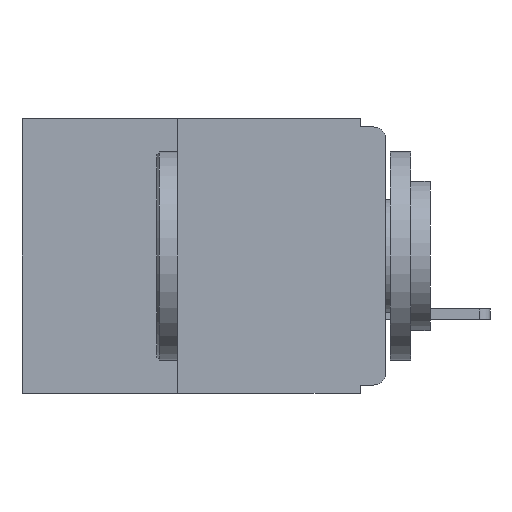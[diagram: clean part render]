
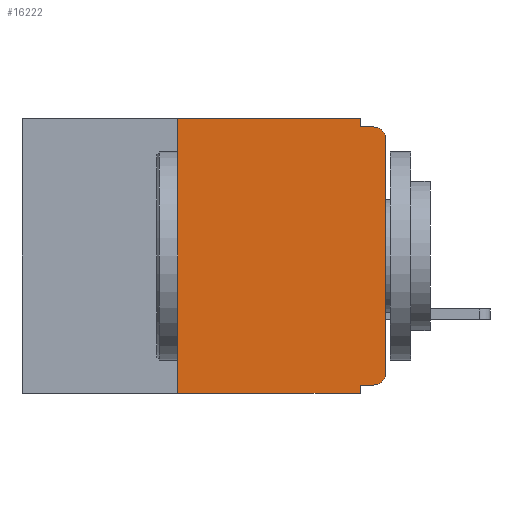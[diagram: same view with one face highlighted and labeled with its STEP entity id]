
A CAD part, left-side view. The second image highlights one B-rep face of the part: STEP entity #16222.
In plain terms, the highlighted planar face has unit normal (-1, 0, 0).
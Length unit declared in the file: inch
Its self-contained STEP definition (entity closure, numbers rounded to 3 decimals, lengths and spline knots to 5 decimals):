
#193 = CARTESIAN_POINT ( 'NONE',  ( 0., 0.25, -0.33 ) ) ;
#539 = VERTEX_POINT ( 'NONE', #2315 ) ;
#827 = DIRECTION ( 'NONE',  ( 0., 0., 1. ) ) ;
#1279 = VERTEX_POINT ( 'NONE', #30754 ) ;
#1551 = CARTESIAN_POINT ( 'NONE',  ( 0., 0.437, 0. ) ) ;
#1604 = VECTOR ( 'NONE', #6091, 39.37008 ) ;
#2132 = CARTESIAN_POINT ( 'NONE',  ( 0., 0., -0.025 ) ) ;
#2315 = CARTESIAN_POINT ( 'NONE',  ( 0., 0.031, -0.33 ) ) ;
#2567 = VERTEX_POINT ( 'NONE', #16467 ) ;
#2939 = ORIENTED_EDGE ( 'NONE', *, *, #4405, .F. ) ;
#4150 = DIRECTION ( 'NONE',  ( 0., -1., 0. ) ) ;
#4205 = LINE ( 'NONE', #1551, #23643 ) ;
#4405 = EDGE_CURVE ( 'NONE', #2567, #15590, #22816, .T. ) ;
#4991 = ORIENTED_EDGE ( 'NONE', *, *, #16368, .T. ) ;
#5085 = CARTESIAN_POINT ( 'NONE',  ( 0., 0.015, -0.305 ) ) ;
#5114 = VECTOR ( 'NONE', #10338, 39.37008 ) ;
#6091 = DIRECTION ( 'NONE',  ( 0., 0., -1. ) ) ;
#6800 = AXIS2_PLACEMENT_3D ( 'NONE', #28515, #13353, #31026 ) ;
#7520 = CARTESIAN_POINT ( 'NONE',  ( 0., 0.015, -0.32 ) ) ;
#7654 = DIRECTION ( 'NONE',  ( 0., 0., -1. ) ) ;
#7661 = ORIENTED_EDGE ( 'NONE', *, *, #28805, .F. ) ;
#7833 = VECTOR ( 'NONE', #26957, 39.37008 ) ;
#9112 = ORIENTED_EDGE ( 'NONE', *, *, #11240, .T. ) ;
#9179 = ORIENTED_EDGE ( 'NONE', *, *, #23349, .T. ) ;
#9200 = LINE ( 'NONE', #13595, #1604 ) ;
#10338 = DIRECTION ( 'NONE',  ( 0., 1., 0. ) ) ;
#10915 = AXIS2_PLACEMENT_3D ( 'NONE', #14170, #31842, #16793 ) ;
#11141 = CARTESIAN_POINT ( 'NONE',  ( 0., 0.031, -0.01 ) ) ;
#11240 = EDGE_CURVE ( 'NONE', #19077, #22179, #11876, .T. ) ;
#11675 = EDGE_CURVE ( 'NONE', #15250, #22444, #25360, .T. ) ;
#11876 = LINE ( 'NONE', #13205, #24597 ) ;
#11890 = ORIENTED_EDGE ( 'NONE', *, *, #26923, .F. ) ;
#12312 = DIRECTION ( 'NONE',  ( 0., -1., 0. ) ) ;
#12396 = EDGE_CURVE ( 'NONE', #22179, #15454, #22551, .T. ) ;
#12964 = LINE ( 'NONE', #19940, #31514 ) ;
#13205 = CARTESIAN_POINT ( 'NONE',  ( 0., 0., 0. ) ) ;
#13302 = EDGE_CURVE ( 'NONE', #15590, #15454, #14511, .T. ) ;
#13353 = DIRECTION ( 'NONE',  ( -1., 0., 0. ) ) ;
#13478 = CARTESIAN_POINT ( 'NONE',  ( 0., 0.25, -0.33 ) ) ;
#13595 = CARTESIAN_POINT ( 'NONE',  ( 0., 0.031, -0.33 ) ) ;
#13956 = DIRECTION ( 'NONE',  ( 0., 0., -1. ) ) ;
#14170 = CARTESIAN_POINT ( 'NONE',  ( 0., 0.437, 0. ) ) ;
#14511 = LINE ( 'NONE', #26842, #7833 ) ;
#15207 = VECTOR ( 'NONE', #13956, 39.37008 ) ;
#15250 = VERTEX_POINT ( 'NONE', #7520 ) ;
#15373 = ORIENTED_EDGE ( 'NONE', *, *, #13302, .F. ) ;
#15454 = VERTEX_POINT ( 'NONE', #18302 ) ;
#15590 = VERTEX_POINT ( 'NONE', #11141 ) ;
#16009 = CARTESIAN_POINT ( 'NONE',  ( 0., 0.031, 0. ) ) ;
#16209 = ORIENTED_EDGE ( 'NONE', *, *, #11675, .F. ) ;
#16222 = ADVANCED_FACE ( 'NONE', ( #22934 ), #31738, .F. ) ;
#16368 = EDGE_CURVE ( 'NONE', #22775, #539, #12964, .T. ) ;
#16467 = CARTESIAN_POINT ( 'NONE',  ( 0., 0.031, 0. ) ) ;
#16793 = DIRECTION ( 'NONE',  ( 0., 0., -1. ) ) ;
#18302 = CARTESIAN_POINT ( 'NONE',  ( 0., 0.015, -0.01 ) ) ;
#19077 = VERTEX_POINT ( 'NONE', #27930 ) ;
#19821 = AXIS2_PLACEMENT_3D ( 'NONE', #5085, #22854, #7654 ) ;
#19940 = CARTESIAN_POINT ( 'NONE',  ( 0., 0.437, -0.33 ) ) ;
#20606 = EDGE_LOOP ( 'NONE', ( #9112, #32207, #15373, #2939, #11890, #7661, #4991, #31195, #16209, #9179 ) ) ;
#22179 = VERTEX_POINT ( 'NONE', #2132 ) ;
#22444 = VERTEX_POINT ( 'NONE', #26093 ) ;
#22551 = CIRCLE ( 'NONE', #6800, 0.015 ) ;
#22750 = CIRCLE ( 'NONE', #19821, 0.015 ) ;
#22775 = VERTEX_POINT ( 'NONE', #193 ) ;
#22816 = LINE ( 'NONE', #16009, #15207 ) ;
#22854 = DIRECTION ( 'NONE',  ( -1., 0., 0. ) ) ;
#22934 = FACE_OUTER_BOUND ( 'NONE', #20606, .T. ) ;
#23349 = EDGE_CURVE ( 'NONE', #15250, #19077, #22750, .T. ) ;
#23443 = DIRECTION ( 'NONE',  ( 0., 0., 1. ) ) ;
#23643 = VECTOR ( 'NONE', #4150, 39.37008 ) ;
#24400 = VECTOR ( 'NONE', #827, 39.37008 ) ;
#24597 = VECTOR ( 'NONE', #23443, 39.37008 ) ;
#25360 = LINE ( 'NONE', #30521, #5114 ) ;
#26093 = CARTESIAN_POINT ( 'NONE',  ( 0., 0.031, -0.32 ) ) ;
#26842 = CARTESIAN_POINT ( 'NONE',  ( 0., 0., -0.01 ) ) ;
#26923 = EDGE_CURVE ( 'NONE', #1279, #2567, #4205, .T. ) ;
#26957 = DIRECTION ( 'NONE',  ( 0., -1., 0. ) ) ;
#27930 = CARTESIAN_POINT ( 'NONE',  ( 0., 0., -0.305 ) ) ;
#28515 = CARTESIAN_POINT ( 'NONE',  ( 0., 0.015, -0.025 ) ) ;
#28805 = EDGE_CURVE ( 'NONE', #22775, #1279, #31030, .T. ) ;
#30521 = CARTESIAN_POINT ( 'NONE',  ( 0., 0., -0.32 ) ) ;
#30555 = EDGE_CURVE ( 'NONE', #22444, #539, #9200, .T. ) ;
#30754 = CARTESIAN_POINT ( 'NONE',  ( 0., 0.25, 0. ) ) ;
#31026 = DIRECTION ( 'NONE',  ( 0., 0., -1. ) ) ;
#31030 = LINE ( 'NONE', #13478, #24400 ) ;
#31195 = ORIENTED_EDGE ( 'NONE', *, *, #30555, .F. ) ;
#31514 = VECTOR ( 'NONE', #12312, 39.37008 ) ;
#31738 = PLANE ( 'NONE',  #10915 ) ;
#31842 = DIRECTION ( 'NONE',  ( 1., 0., 0. ) ) ;
#32207 = ORIENTED_EDGE ( 'NONE', *, *, #12396, .T. ) ;
